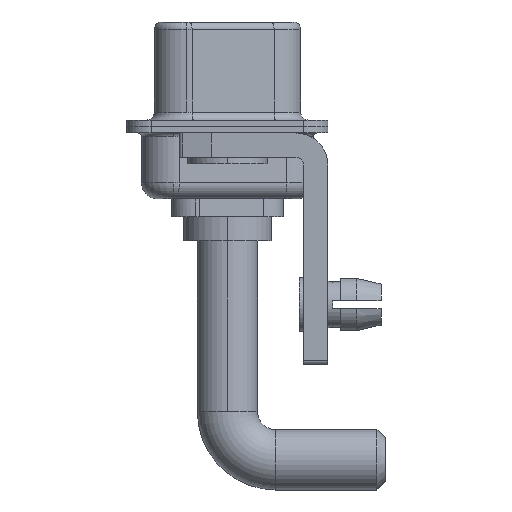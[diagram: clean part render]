
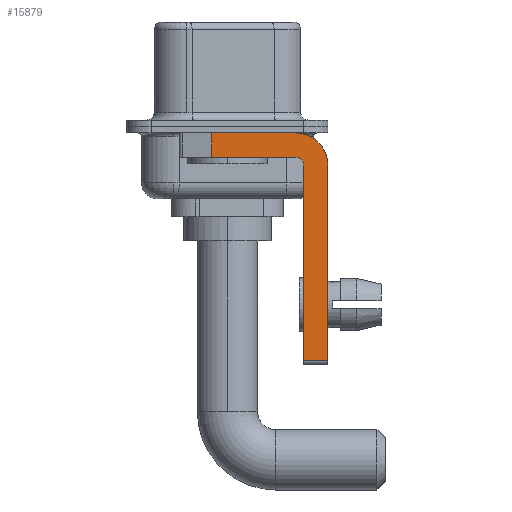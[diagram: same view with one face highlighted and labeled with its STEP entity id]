
A CAD part, left-side view. The second image highlights one B-rep face of the part: STEP entity #15879.
In plain terms, the highlighted planar face has unit normal (-1, 0, 0).
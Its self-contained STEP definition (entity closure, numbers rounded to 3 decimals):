
#157 = ORIENTED_EDGE ( 'NONE', *, *, #10043, .F. ) ;
#294 = CARTESIAN_POINT ( 'NONE',  ( -2.9, 3., -0.4 ) ) ;
#376 = VECTOR ( 'NONE', #8882, 1000. ) ;
#457 = EDGE_LOOP ( 'NONE', ( #12192, #11450, #10661, #14381, #9940, #529, #1414, #157 ) ) ;
#529 = ORIENTED_EDGE ( 'NONE', *, *, #1487, .T. ) ;
#742 = DIRECTION ( 'NONE',  ( 1., 0., 0. ) ) ;
#1414 = ORIENTED_EDGE ( 'NONE', *, *, #6529, .F. ) ;
#1487 = EDGE_CURVE ( 'NONE', #18013, #15919, #17711, .T. ) ;
#1970 = EDGE_CURVE ( 'NONE', #2023, #2692, #14968, .T. ) ;
#2023 = VERTEX_POINT ( 'NONE', #16302 ) ;
#2692 = VERTEX_POINT ( 'NONE', #15314 ) ;
#2732 = CARTESIAN_POINT ( 'NONE',  ( -2.9, -4.75, -14.8 ) ) ;
#3028 = CARTESIAN_POINT ( 'NONE',  ( -2.9, -6.25, -2.4 ) ) ;
#3522 = AXIS2_PLACEMENT_3D ( 'NONE', #7559, #742, #9236 ) ;
#3568 = DIRECTION ( 'NONE',  ( 0., 0., 1. ) ) ;
#4302 = CARTESIAN_POINT ( 'NONE',  ( -2.9, 0.978, -0.4 ) ) ;
#4731 = CARTESIAN_POINT ( 'NONE',  ( -2.9, -4.25, -14.55 ) ) ;
#4896 = CARTESIAN_POINT ( 'NONE',  ( -2.9, -4.25, -2.4 ) ) ;
#5136 = EDGE_CURVE ( 'NONE', #2692, #10885, #18474, .T. ) ;
#6335 = CARTESIAN_POINT ( 'NONE',  ( -2.9, 0.978, -1.9 ) ) ;
#6529 = EDGE_CURVE ( 'NONE', #7074, #15919, #10002, .T. ) ;
#6917 = AXIS2_PLACEMENT_3D ( 'NONE', #4896, #7686, #3568 ) ;
#7074 = VERTEX_POINT ( 'NONE', #3028 ) ;
#7540 = VERTEX_POINT ( 'NONE', #10585 ) ;
#7559 = CARTESIAN_POINT ( 'NONE',  ( -2.9, -4.25, -2.4 ) ) ;
#7662 = LINE ( 'NONE', #294, #376 ) ;
#7686 = DIRECTION ( 'NONE',  ( -1., 0., 0. ) ) ;
#8436 = DIRECTION ( 'NONE',  ( 0., 0., 1. ) ) ;
#8669 = EDGE_CURVE ( 'NONE', #13667, #7540, #7662, .T. ) ;
#8882 = DIRECTION ( 'NONE',  ( 0., -1., 0. ) ) ;
#9133 = VECTOR ( 'NONE', #16358, 1000. ) ;
#9236 = DIRECTION ( 'NONE',  ( 0., 0., -1. ) ) ;
#9255 = VECTOR ( 'NONE', #16732, 1000. ) ;
#9339 = VECTOR ( 'NONE', #8436, 1000. ) ;
#9520 = LINE ( 'NONE', #6335, #9133 ) ;
#9940 = ORIENTED_EDGE ( 'NONE', *, *, #10965, .F. ) ;
#10002 = LINE ( 'NONE', #18402, #9255 ) ;
#10043 = EDGE_CURVE ( 'NONE', #7540, #7074, #17123, .T. ) ;
#10285 = AXIS2_PLACEMENT_3D ( 'NONE', #12082, #10496, #11811 ) ;
#10391 = CARTESIAN_POINT ( 'NONE',  ( -2.9, -6.25, -14.55 ) ) ;
#10496 = DIRECTION ( 'NONE',  ( 1., 0., 0. ) ) ;
#10585 = CARTESIAN_POINT ( 'NONE',  ( -2.9, -4.25, -0.4 ) ) ;
#10661 = ORIENTED_EDGE ( 'NONE', *, *, #5136, .F. ) ;
#10885 = VERTEX_POINT ( 'NONE', #13019 ) ;
#10965 = EDGE_CURVE ( 'NONE', #18013, #2023, #15545, .T. ) ;
#11450 = ORIENTED_EDGE ( 'NONE', *, *, #14074, .T. ) ;
#11811 = DIRECTION ( 'NONE',  ( 0., 0., -1. ) ) ;
#11963 = FACE_OUTER_BOUND ( 'NONE', #457, .T. ) ;
#12082 = CARTESIAN_POINT ( 'NONE',  ( -2.9, -4.25, -2.4 ) ) ;
#12192 = ORIENTED_EDGE ( 'NONE', *, *, #8669, .F. ) ;
#12679 = CARTESIAN_POINT ( 'NONE',  ( -2.9, -4.75, -14.55 ) ) ;
#12780 = DIRECTION ( 'NONE',  ( 0., 1., 0. ) ) ;
#13019 = CARTESIAN_POINT ( 'NONE',  ( -2.9, 0.978, -1.9 ) ) ;
#13403 = VECTOR ( 'NONE', #12780, 1000. ) ;
#13667 = VERTEX_POINT ( 'NONE', #4302 ) ;
#14074 = EDGE_CURVE ( 'NONE', #13667, #10885, #9520, .T. ) ;
#14381 = ORIENTED_EDGE ( 'NONE', *, *, #1970, .F. ) ;
#14968 = CIRCLE ( 'NONE', #6917, 0.5 ) ;
#15314 = CARTESIAN_POINT ( 'NONE',  ( -2.9, -4.25, -1.9 ) ) ;
#15545 = LINE ( 'NONE', #2732, #9339 ) ;
#15770 = CARTESIAN_POINT ( 'NONE',  ( -2.9, -4.25, -1.9 ) ) ;
#15879 = ADVANCED_FACE ( 'NONE', ( #11963 ), #17653, .F. ) ;
#15919 = VERTEX_POINT ( 'NONE', #10391 ) ;
#16134 = DIRECTION ( 'NONE',  ( 0., -1., 0. ) ) ;
#16302 = CARTESIAN_POINT ( 'NONE',  ( -2.9, -4.75, -2.4 ) ) ;
#16358 = DIRECTION ( 'NONE',  ( 0., 0., -1. ) ) ;
#16732 = DIRECTION ( 'NONE',  ( 0., 0., -1. ) ) ;
#17123 = CIRCLE ( 'NONE', #10285, 2. ) ;
#17653 = PLANE ( 'NONE',  #3522 ) ;
#17711 = LINE ( 'NONE', #4731, #18144 ) ;
#18013 = VERTEX_POINT ( 'NONE', #12679 ) ;
#18144 = VECTOR ( 'NONE', #16134, 1000. ) ;
#18402 = CARTESIAN_POINT ( 'NONE',  ( -2.9, -6.25, -2.4 ) ) ;
#18474 = LINE ( 'NONE', #15770, #13403 ) ;
